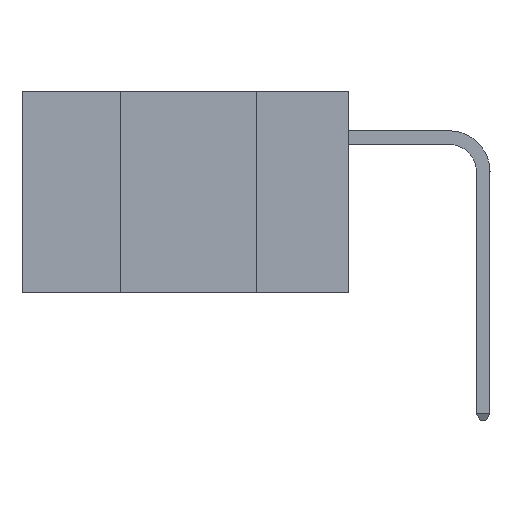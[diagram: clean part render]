
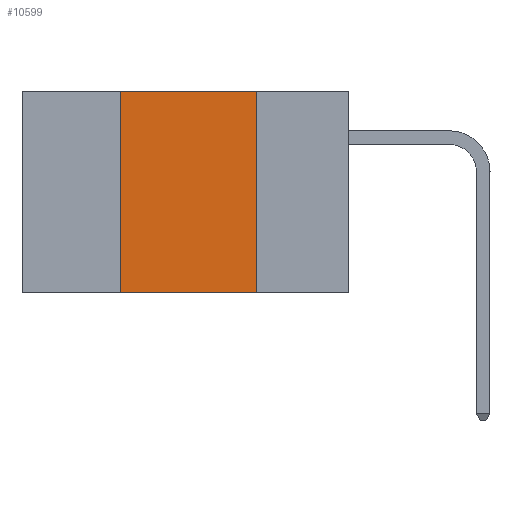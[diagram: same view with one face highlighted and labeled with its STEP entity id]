
A CAD part, left-side view. The second image highlights one B-rep face of the part: STEP entity #10599.
In plain terms, the highlighted planar face has unit normal (-1, 0, 0).
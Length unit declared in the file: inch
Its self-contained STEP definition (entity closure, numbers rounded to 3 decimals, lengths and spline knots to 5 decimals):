
#106 = EDGE_CURVE ( 'NONE', #6527, #2241, #6713, .T. ) ;
#113 = CARTESIAN_POINT ( 'NONE',  ( 0., 0.17, 0. ) ) ;
#167 = DIRECTION ( 'NONE',  ( 0., -1., 0. ) ) ;
#348 = CARTESIAN_POINT ( 'NONE',  ( 0., 0.6, 0. ) ) ;
#378 = DIRECTION ( 'NONE',  ( 1., 0., 0. ) ) ;
#386 = AXIS2_PLACEMENT_3D ( 'NONE', #8519, #378, #7342 ) ;
#1137 = LINE ( 'NONE', #6810, #5130 ) ;
#1184 = CARTESIAN_POINT ( 'NONE',  ( 0., 0.6, -0.37 ) ) ;
#1691 = CARTESIAN_POINT ( 'NONE',  ( 0., 0.42, 0. ) ) ;
#1743 = CARTESIAN_POINT ( 'NONE',  ( 0., 0.17, -0.37 ) ) ;
#2024 = VECTOR ( 'NONE', #4820, 39.37008 ) ;
#2241 = VERTEX_POINT ( 'NONE', #1743 ) ;
#2527 = EDGE_CURVE ( 'NONE', #6748, #10227, #10260, .T. ) ;
#3797 = LINE ( 'NONE', #4788, #2024 ) ;
#3978 = ORIENTED_EDGE ( 'NONE', *, *, #8401, .F. ) ;
#3983 = EDGE_LOOP ( 'NONE', ( #10605, #5233, #3978, #11320 ) ) ;
#4424 = VECTOR ( 'NONE', #167, 39.37008 ) ;
#4788 = CARTESIAN_POINT ( 'NONE',  ( 0., 0.42, 0. ) ) ;
#4820 = DIRECTION ( 'NONE',  ( 0., 0., 1. ) ) ;
#4975 = PLANE ( 'NONE',  #386 ) ;
#5130 = VECTOR ( 'NONE', #6106, 39.37008 ) ;
#5233 = ORIENTED_EDGE ( 'NONE', *, *, #2527, .F. ) ;
#6106 = DIRECTION ( 'NONE',  ( 0., 0., -1. ) ) ;
#6527 = VERTEX_POINT ( 'NONE', #8001 ) ;
#6713 = LINE ( 'NONE', #1184, #4424 ) ;
#6748 = VERTEX_POINT ( 'NONE', #1691 ) ;
#6810 = CARTESIAN_POINT ( 'NONE',  ( 0., 0.17, 0. ) ) ;
#7073 = VECTOR ( 'NONE', #10885, 39.37008 ) ;
#7342 = DIRECTION ( 'NONE',  ( 0., 0., -1. ) ) ;
#8001 = CARTESIAN_POINT ( 'NONE',  ( 0., 0.42, -0.37 ) ) ;
#8401 = EDGE_CURVE ( 'NONE', #6527, #6748, #3797, .T. ) ;
#8519 = CARTESIAN_POINT ( 'NONE',  ( 0., 0.6, 0. ) ) ;
#10108 = FACE_OUTER_BOUND ( 'NONE', #3983, .T. ) ;
#10227 = VERTEX_POINT ( 'NONE', #113 ) ;
#10260 = LINE ( 'NONE', #348, #7073 ) ;
#10599 = ADVANCED_FACE ( 'NONE', ( #10108 ), #4975, .F. ) ;
#10605 = ORIENTED_EDGE ( 'NONE', *, *, #11208, .F. ) ;
#10885 = DIRECTION ( 'NONE',  ( 0., -1., 0. ) ) ;
#11208 = EDGE_CURVE ( 'NONE', #10227, #2241, #1137, .T. ) ;
#11320 = ORIENTED_EDGE ( 'NONE', *, *, #106, .T. ) ;
